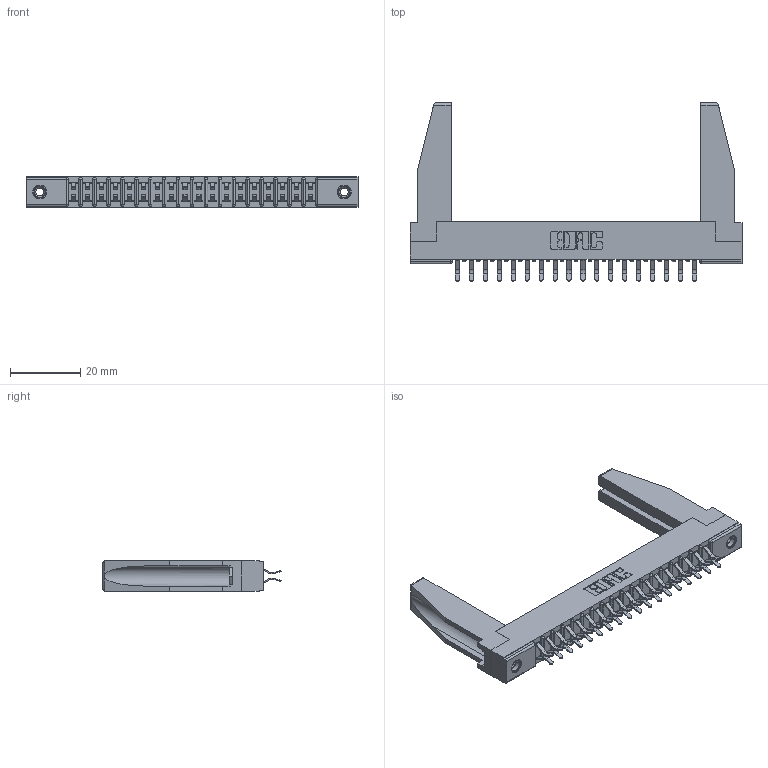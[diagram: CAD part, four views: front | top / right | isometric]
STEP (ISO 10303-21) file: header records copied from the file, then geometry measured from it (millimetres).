
FILE_DESCRIPTION (( 'STEP AP203' ), '1' );
FILE_NAME ('307-036-556-278.STEP', '2019-09-06T03:48:05', ( '' ), ( '' ), 'SwSTEP 2.0', 'SolidWorks 2016', '' );
FILE_SCHEMA (( 'CONFIG_CONTROL_DESIGN' ));
Length unit declared in the file: inch
Products named in the file (5): 307 Part_.156 Dia Mounting Holes; 307-290-001_556; 307-220-078; 345-250-001_345-250-001-102; 307-036-556-278
Assembly tree (41 placements, depth 2):
  307-036-556-278
    307 Part_.156 Dia Mounting Holes
    307-290-001_556  x36
    307-220-078  x2
    345-250-001_345-250-001-102  x2
Bounding box: 94.34 x 50.67 x 8.71 mm (x, y, z)
Volume: 10157.8 mm3; surface area: 14467.4 mm2
Topology: 41 solids, 41 shells, 2067 faces, 5765 edges, 3734 vertices
Faces by surface type: plane 1342, cylinder 671, sphere 38, cone 12, torus 4
Entity records: 21509 total; most frequent: CARTESIAN_POINT 3536, ORIENTED_EDGE 3460, DIRECTION 3428, EDGE_CURVE 1730, VECTOR 1320, LINE 1320, VERTEX_POINT 1120, AXIS2_PLACEMENT_3D 1054
